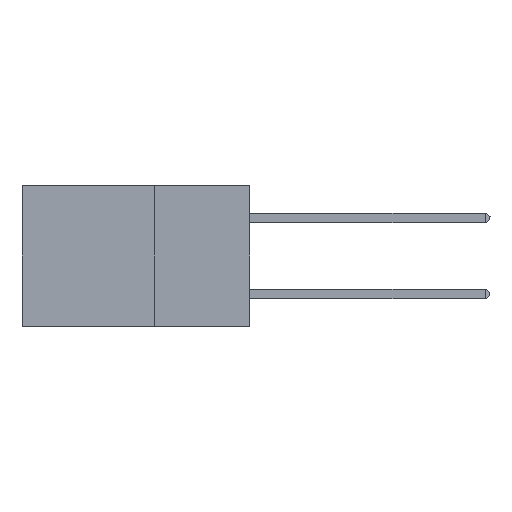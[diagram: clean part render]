
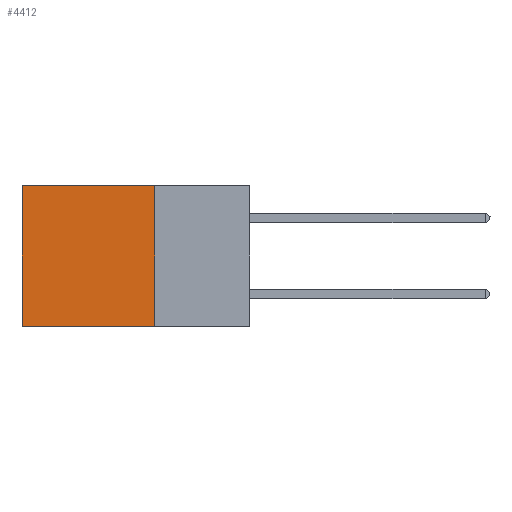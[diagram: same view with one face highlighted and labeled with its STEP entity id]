
A CAD part, left-side view. The second image highlights one B-rep face of the part: STEP entity #4412.
In plain terms, the highlighted planar face has unit normal (-1, 0, 0).
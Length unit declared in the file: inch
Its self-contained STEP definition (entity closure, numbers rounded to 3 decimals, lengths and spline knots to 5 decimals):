
#126 = DIRECTION ( 'NONE',  ( 1., 0., 0. ) ) ;
#1945 = LINE ( 'NONE', #16794, #19446 ) ;
#2609 = EDGE_CURVE ( 'NONE', #4645, #15599, #1945, .T. ) ;
#3189 = CARTESIAN_POINT ( 'NONE',  ( 0.2875, 0.25, -0.37 ) ) ;
#4412 = ADVANCED_FACE ( 'NONE', ( #17928 ), #18722, .F. ) ;
#4645 = VERTEX_POINT ( 'NONE', #10776 ) ;
#4810 = ORIENTED_EDGE ( 'NONE', *, *, #2609, .F. ) ;
#4962 = DIRECTION ( 'NONE',  ( 0., 0., -1. ) ) ;
#6626 = DIRECTION ( 'NONE',  ( 0., 0., -1. ) ) ;
#6889 = DIRECTION ( 'NONE',  ( 0., 1., 0. ) ) ;
#7616 = CARTESIAN_POINT ( 'NONE',  ( 0.2875, 0.6, 0. ) ) ;
#9194 = ORIENTED_EDGE ( 'NONE', *, *, #20168, .T. ) ;
#9319 = LINE ( 'NONE', #20458, #21783 ) ;
#10776 = CARTESIAN_POINT ( 'NONE',  ( 0.2875, 0.25, 0. ) ) ;
#11962 = DIRECTION ( 'NONE',  ( 0., 0., -1. ) ) ;
#12274 = LINE ( 'NONE', #21914, #16236 ) ;
#12955 = ORIENTED_EDGE ( 'NONE', *, *, #18587, .F. ) ;
#14980 = VERTEX_POINT ( 'NONE', #20228 ) ;
#15195 = EDGE_LOOP ( 'NONE', ( #16831, #12955, #4810, #9194 ) ) ;
#15599 = VERTEX_POINT ( 'NONE', #3189 ) ;
#16236 = VECTOR ( 'NONE', #6626, 39.37008 ) ;
#16591 = VECTOR ( 'NONE', #19886, 39.37008 ) ;
#16794 = CARTESIAN_POINT ( 'NONE',  ( 0.2875, 0.25, 0. ) ) ;
#16831 = ORIENTED_EDGE ( 'NONE', *, *, #17751, .T. ) ;
#16943 = AXIS2_PLACEMENT_3D ( 'NONE', #20414, #126, #11962 ) ;
#17481 = VERTEX_POINT ( 'NONE', #7616 ) ;
#17751 = EDGE_CURVE ( 'NONE', #17481, #14980, #12274, .T. ) ;
#17928 = FACE_OUTER_BOUND ( 'NONE', #15195, .T. ) ;
#18193 = CARTESIAN_POINT ( 'NONE',  ( 0.2875, 0.25, 0. ) ) ;
#18587 = EDGE_CURVE ( 'NONE', #15599, #14980, #9319, .T. ) ;
#18722 = PLANE ( 'NONE',  #16943 ) ;
#19446 = VECTOR ( 'NONE', #4962, 39.37008 ) ;
#19886 = DIRECTION ( 'NONE',  ( 0., 1., 0. ) ) ;
#20059 = LINE ( 'NONE', #18193, #16591 ) ;
#20168 = EDGE_CURVE ( 'NONE', #4645, #17481, #20059, .T. ) ;
#20228 = CARTESIAN_POINT ( 'NONE',  ( 0.2875, 0.6, -0.37 ) ) ;
#20414 = CARTESIAN_POINT ( 'NONE',  ( 0.2875, 0.25, 0. ) ) ;
#20458 = CARTESIAN_POINT ( 'NONE',  ( 0.2875, 0.25, -0.37 ) ) ;
#21783 = VECTOR ( 'NONE', #6889, 39.37008 ) ;
#21914 = CARTESIAN_POINT ( 'NONE',  ( 0.2875, 0.6, 0. ) ) ;
